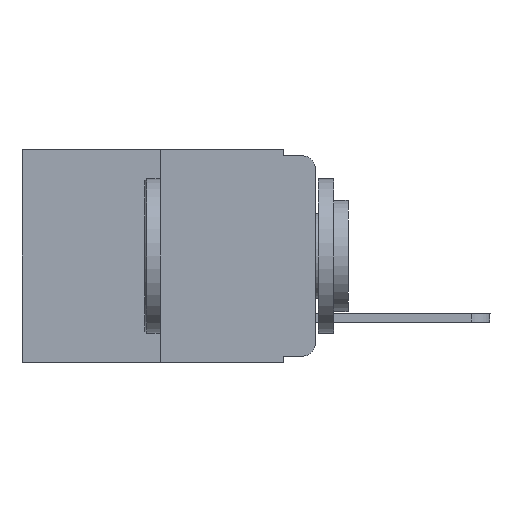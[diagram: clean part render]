
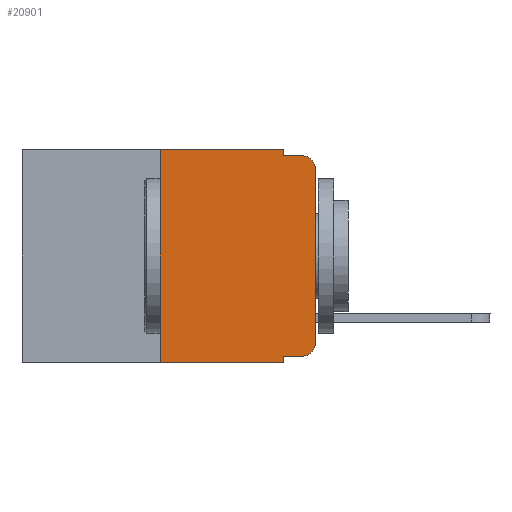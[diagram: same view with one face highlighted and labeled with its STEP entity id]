
A CAD part, left-side view. The second image highlights one B-rep face of the part: STEP entity #20901.
In plain terms, the highlighted planar face has unit normal (-1, 0, 0).
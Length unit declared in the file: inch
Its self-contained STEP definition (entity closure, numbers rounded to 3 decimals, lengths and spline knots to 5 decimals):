
#234 = CARTESIAN_POINT ( 'NONE',  ( 0., 0., -0.03 ) ) ;
#326 = VERTEX_POINT ( 'NONE', #7087 ) ;
#671 = DIRECTION ( 'NONE',  ( 1., 0., 0. ) ) ;
#1209 = VECTOR ( 'NONE', #7925, 39.37008 ) ;
#2411 = CARTESIAN_POINT ( 'NONE',  ( 0., 0.051, 0. ) ) ;
#2859 = VECTOR ( 'NONE', #12221, 39.37008 ) ;
#3960 = CARTESIAN_POINT ( 'NONE',  ( 0., 0.473, -0.343 ) ) ;
#4318 = CARTESIAN_POINT ( 'NONE',  ( 0., 0.051, -0.01 ) ) ;
#4330 = CARTESIAN_POINT ( 'NONE',  ( 0., 0.25, 0. ) ) ;
#4583 = AXIS2_PLACEMENT_3D ( 'NONE', #8043, #25743, #9905 ) ;
#4695 = EDGE_CURVE ( 'NONE', #13129, #16999, #18378, .T. ) ;
#5523 = CARTESIAN_POINT ( 'NONE',  ( 0., 0., -0.313 ) ) ;
#5600 = ORIENTED_EDGE ( 'NONE', *, *, #23844, .T. ) ;
#5645 = LINE ( 'NONE', #10030, #1209 ) ;
#6812 = DIRECTION ( 'NONE',  ( 0., -1., 0. ) ) ;
#7087 = CARTESIAN_POINT ( 'NONE',  ( 0., 0.051, -0.333 ) ) ;
#7925 = DIRECTION ( 'NONE',  ( 0., -1., 0. ) ) ;
#8043 = CARTESIAN_POINT ( 'NONE',  ( 0., 0.02, -0.03 ) ) ;
#8128 = CARTESIAN_POINT ( 'NONE',  ( 0., 0.051, -0.333 ) ) ;
#8289 = VECTOR ( 'NONE', #22092, 39.37008 ) ;
#8693 = DIRECTION ( 'NONE',  ( 0., 0., -1. ) ) ;
#8823 = VERTEX_POINT ( 'NONE', #14919 ) ;
#9056 = ORIENTED_EDGE ( 'NONE', *, *, #18567, .F. ) ;
#9064 = EDGE_CURVE ( 'NONE', #18766, #22057, #10032, .T. ) ;
#9137 = EDGE_CURVE ( 'NONE', #9237, #25967, #22902, .T. ) ;
#9237 = VERTEX_POINT ( 'NONE', #25487 ) ;
#9831 = DIRECTION ( 'NONE',  ( -1., 0., 0. ) ) ;
#9905 = DIRECTION ( 'NONE',  ( 0., 0., -1. ) ) ;
#10030 = CARTESIAN_POINT ( 'NONE',  ( 0., 0.473, 0. ) ) ;
#10032 = LINE ( 'NONE', #10579, #25381 ) ;
#10053 = ORIENTED_EDGE ( 'NONE', *, *, #4695, .T. ) ;
#10116 = VECTOR ( 'NONE', #24721, 39.37008 ) ;
#10145 = VECTOR ( 'NONE', #25584, 39.37008 ) ;
#10579 = CARTESIAN_POINT ( 'NONE',  ( 0., 0.051, -0.01 ) ) ;
#10777 = VERTEX_POINT ( 'NONE', #4330 ) ;
#10919 = CARTESIAN_POINT ( 'NONE',  ( 0., 0.051, -0.343 ) ) ;
#11031 = AXIS2_PLACEMENT_3D ( 'NONE', #21839, #9831, #19635 ) ;
#11064 = LINE ( 'NONE', #25324, #10145 ) ;
#11758 = ORIENTED_EDGE ( 'NONE', *, *, #13248, .F. ) ;
#12221 = DIRECTION ( 'NONE',  ( 0., 0., -1. ) ) ;
#12290 = ORIENTED_EDGE ( 'NONE', *, *, #12853, .T. ) ;
#12356 = LINE ( 'NONE', #8128, #8289 ) ;
#12429 = CARTESIAN_POINT ( 'NONE',  ( 0., 0.25, 0. ) ) ;
#12853 = EDGE_CURVE ( 'NONE', #16999, #19156, #11064, .T. ) ;
#13129 = VERTEX_POINT ( 'NONE', #25820 ) ;
#13248 = EDGE_CURVE ( 'NONE', #8823, #18766, #22689, .T. ) ;
#13622 = AXIS2_PLACEMENT_3D ( 'NONE', #18962, #671, #8693 ) ;
#13969 = CARTESIAN_POINT ( 'NONE',  ( 0., 0.051, 0. ) ) ;
#14919 = CARTESIAN_POINT ( 'NONE',  ( 0., 0.051, 0. ) ) ;
#15908 = DIRECTION ( 'NONE',  ( 0., -1., 0. ) ) ;
#15925 = EDGE_CURVE ( 'NONE', #326, #25967, #24412, .T. ) ;
#16247 = VECTOR ( 'NONE', #16446, 39.37008 ) ;
#16308 = ORIENTED_EDGE ( 'NONE', *, *, #9064, .F. ) ;
#16442 = ORIENTED_EDGE ( 'NONE', *, *, #15925, .F. ) ;
#16446 = DIRECTION ( 'NONE',  ( 0., 0., -1. ) ) ;
#16999 = VERTEX_POINT ( 'NONE', #5523 ) ;
#17699 = EDGE_CURVE ( 'NONE', #10777, #8823, #5645, .T. ) ;
#18064 = CIRCLE ( 'NONE', #4583, 0.02 ) ;
#18378 = CIRCLE ( 'NONE', #11031, 0.02 ) ;
#18567 = EDGE_CURVE ( 'NONE', #9237, #10777, #20163, .T. ) ;
#18766 = VERTEX_POINT ( 'NONE', #4318 ) ;
#18962 = CARTESIAN_POINT ( 'NONE',  ( 0., 0.473, 0. ) ) ;
#19156 = VERTEX_POINT ( 'NONE', #234 ) ;
#19539 = ORIENTED_EDGE ( 'NONE', *, *, #23800, .T. ) ;
#19635 = DIRECTION ( 'NONE',  ( 0., 0., -1. ) ) ;
#20163 = LINE ( 'NONE', #12429, #10116 ) ;
#20901 = ADVANCED_FACE ( 'NONE', ( #24581 ), #24844, .F. ) ;
#21203 = ORIENTED_EDGE ( 'NONE', *, *, #9137, .T. ) ;
#21839 = CARTESIAN_POINT ( 'NONE',  ( 0., 0.02, -0.313 ) ) ;
#22057 = VERTEX_POINT ( 'NONE', #22600 ) ;
#22092 = DIRECTION ( 'NONE',  ( 0., -1., 0. ) ) ;
#22600 = CARTESIAN_POINT ( 'NONE',  ( 0., 0.02, -0.01 ) ) ;
#22689 = LINE ( 'NONE', #13969, #2859 ) ;
#22882 = EDGE_LOOP ( 'NONE', ( #12290, #19539, #16308, #11758, #24185, #9056, #21203, #16442, #5600, #10053 ) ) ;
#22902 = LINE ( 'NONE', #3960, #25988 ) ;
#23800 = EDGE_CURVE ( 'NONE', #19156, #22057, #18064, .T. ) ;
#23844 = EDGE_CURVE ( 'NONE', #326, #13129, #12356, .T. ) ;
#24185 = ORIENTED_EDGE ( 'NONE', *, *, #17699, .F. ) ;
#24412 = LINE ( 'NONE', #2411, #16247 ) ;
#24581 = FACE_OUTER_BOUND ( 'NONE', #22882, .T. ) ;
#24721 = DIRECTION ( 'NONE',  ( 0., 0., 1. ) ) ;
#24844 = PLANE ( 'NONE',  #13622 ) ;
#25324 = CARTESIAN_POINT ( 'NONE',  ( 0., 0., 0. ) ) ;
#25381 = VECTOR ( 'NONE', #6812, 39.37008 ) ;
#25487 = CARTESIAN_POINT ( 'NONE',  ( 0., 0.25, -0.343 ) ) ;
#25584 = DIRECTION ( 'NONE',  ( 0., 0., 1. ) ) ;
#25743 = DIRECTION ( 'NONE',  ( -1., 0., 0. ) ) ;
#25820 = CARTESIAN_POINT ( 'NONE',  ( 0., 0.02, -0.333 ) ) ;
#25967 = VERTEX_POINT ( 'NONE', #10919 ) ;
#25988 = VECTOR ( 'NONE', #15908, 39.37008 ) ;
